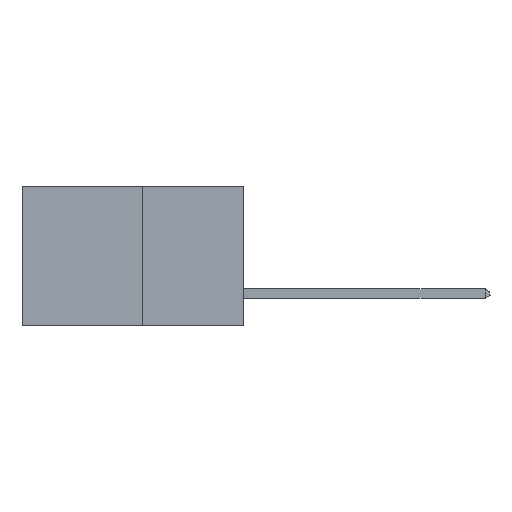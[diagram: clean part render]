
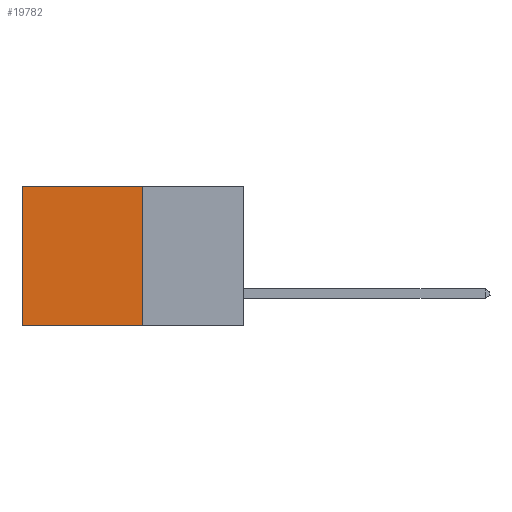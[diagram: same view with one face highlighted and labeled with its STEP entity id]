
A CAD part, left-side view. The second image highlights one B-rep face of the part: STEP entity #19782.
In plain terms, the highlighted planar face has unit normal (-1, 0, 0).
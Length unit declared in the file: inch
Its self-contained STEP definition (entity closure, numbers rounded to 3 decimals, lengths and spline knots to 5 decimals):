
#891 = CARTESIAN_POINT ( 'NONE',  ( 0.277, 0.27, -0.37 ) ) ;
#2252 = VECTOR ( 'NONE', #10811, 39.37008 ) ;
#2505 = CARTESIAN_POINT ( 'NONE',  ( 0.277, 0.27, -0.37 ) ) ;
#3432 = VERTEX_POINT ( 'NONE', #22276 ) ;
#4412 = DIRECTION ( 'NONE',  ( 0., 0., -1. ) ) ;
#4945 = EDGE_LOOP ( 'NONE', ( #7808, #10445, #8994, #13717 ) ) ;
#5419 = VECTOR ( 'NONE', #5610, 39.37008 ) ;
#5610 = DIRECTION ( 'NONE',  ( 0., 0., -1. ) ) ;
#6047 = VERTEX_POINT ( 'NONE', #12642 ) ;
#6355 = DIRECTION ( 'NONE',  ( 0., 1., 0. ) ) ;
#7308 = EDGE_CURVE ( 'NONE', #11365, #3432, #21381, .T. ) ;
#7808 = ORIENTED_EDGE ( 'NONE', *, *, #22165, .T. ) ;
#8228 = CARTESIAN_POINT ( 'NONE',  ( 0.277, 0.27, 0. ) ) ;
#8934 = CARTESIAN_POINT ( 'NONE',  ( 0.277, 0.27, -0.37 ) ) ;
#8994 = ORIENTED_EDGE ( 'NONE', *, *, #23869, .F. ) ;
#9685 = CARTESIAN_POINT ( 'NONE',  ( 0.277, 0.27, 0. ) ) ;
#10445 = ORIENTED_EDGE ( 'NONE', *, *, #20810, .F. ) ;
#10811 = DIRECTION ( 'NONE',  ( 0., 1., 0. ) ) ;
#11365 = VERTEX_POINT ( 'NONE', #9685 ) ;
#11872 = PLANE ( 'NONE',  #13184 ) ;
#12327 = LINE ( 'NONE', #20773, #17254 ) ;
#12642 = CARTESIAN_POINT ( 'NONE',  ( 0.277, 0.59, -0.37 ) ) ;
#13171 = VERTEX_POINT ( 'NONE', #891 ) ;
#13184 = AXIS2_PLACEMENT_3D ( 'NONE', #2505, #15586, #4412 ) ;
#13717 = ORIENTED_EDGE ( 'NONE', *, *, #7308, .T. ) ;
#14882 = CARTESIAN_POINT ( 'NONE',  ( 0.277, 0.59, -0.37 ) ) ;
#15586 = DIRECTION ( 'NONE',  ( 1., 0., 0. ) ) ;
#16600 = VECTOR ( 'NONE', #6355, 39.37008 ) ;
#17127 = FACE_OUTER_BOUND ( 'NONE', #4945, .T. ) ;
#17141 = LINE ( 'NONE', #8934, #2252 ) ;
#17254 = VECTOR ( 'NONE', #17255, 39.37008 ) ;
#17255 = DIRECTION ( 'NONE',  ( 0., 0., -1. ) ) ;
#19042 = LINE ( 'NONE', #14882, #5419 ) ;
#19782 = ADVANCED_FACE ( 'NONE', ( #17127 ), #11872, .F. ) ;
#20773 = CARTESIAN_POINT ( 'NONE',  ( 0.277, 0.27, -0.37 ) ) ;
#20810 = EDGE_CURVE ( 'NONE', #13171, #6047, #17141, .T. ) ;
#21381 = LINE ( 'NONE', #8228, #16600 ) ;
#22165 = EDGE_CURVE ( 'NONE', #3432, #6047, #19042, .T. ) ;
#22276 = CARTESIAN_POINT ( 'NONE',  ( 0.277, 0.59, 0. ) ) ;
#23869 = EDGE_CURVE ( 'NONE', #11365, #13171, #12327, .T. ) ;
